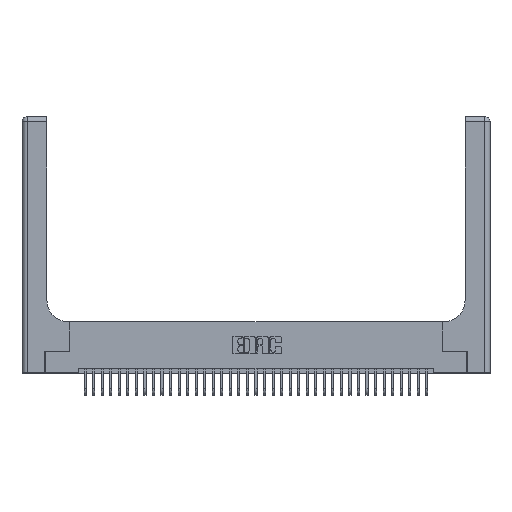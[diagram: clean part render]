
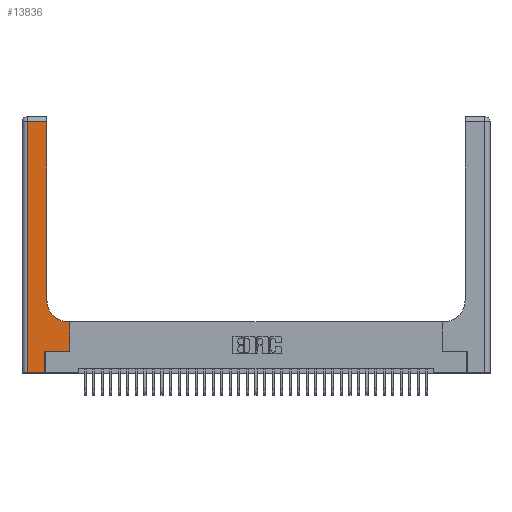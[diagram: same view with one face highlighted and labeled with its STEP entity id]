
A CAD part, top view. The second image highlights one B-rep face of the part: STEP entity #13836.
In plain terms, the highlighted planar face has unit normal (0, 0, 1).
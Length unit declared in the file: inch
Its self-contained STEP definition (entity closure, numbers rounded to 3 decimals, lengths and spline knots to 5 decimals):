
#335 = DIRECTION ( 'NONE',  ( 0., 1., 0. ) ) ;
#1182 = EDGE_LOOP ( 'NONE', ( #3528, #18645, #12930, #21307, #23895, #11593, #5812, #29034, #10288 ) ) ;
#1398 = EDGE_CURVE ( 'NONE', #20830, #19128, #17154, .T. ) ;
#1920 = LINE ( 'NONE', #32527, #17076 ) ;
#3303 = LINE ( 'NONE', #16678, #31379 ) ;
#3528 = ORIENTED_EDGE ( 'NONE', *, *, #5199, .T. ) ;
#5199 = EDGE_CURVE ( 'NONE', #33645, #21898, #26045, .T. ) ;
#5226 = DIRECTION ( 'NONE',  ( 0., -1., 0. ) ) ;
#5538 = VERTEX_POINT ( 'NONE', #17578 ) ;
#5812 = ORIENTED_EDGE ( 'NONE', *, *, #19766, .T. ) ;
#5945 = LINE ( 'NONE', #28538, #26597 ) ;
#6381 = CARTESIAN_POINT ( 'NONE',  ( 0.2915, 2.94, 0.37 ) ) ;
#8155 = DIRECTION ( 'NONE',  ( -1., 0., 0. ) ) ;
#9908 = CARTESIAN_POINT ( 'NONE',  ( 0.5415, 0.85, 0.37 ) ) ;
#10036 = EDGE_CURVE ( 'NONE', #13771, #20830, #5945, .T. ) ;
#10288 = ORIENTED_EDGE ( 'NONE', *, *, #23283, .T. ) ;
#10390 = CARTESIAN_POINT ( 'NONE',  ( 0.2915, 0.6, 0.37 ) ) ;
#11514 = DIRECTION ( 'NONE',  ( 1., 0., 0. ) ) ;
#11593 = ORIENTED_EDGE ( 'NONE', *, *, #1398, .T. ) ;
#12111 = DIRECTION ( 'NONE',  ( 0., 1., 0. ) ) ;
#12151 = VECTOR ( 'NONE', #12111, 39.37008 ) ;
#12765 = DIRECTION ( 'NONE',  ( 1., 0., 0. ) ) ;
#12930 = ORIENTED_EDGE ( 'NONE', *, *, #18725, .T. ) ;
#13298 = CARTESIAN_POINT ( 'NONE',  ( 0.2915, 3., 0.37 ) ) ;
#13396 = CARTESIAN_POINT ( 'NONE',  ( 0.269, 0., 0.37 ) ) ;
#13771 = VERTEX_POINT ( 'NONE', #13396 ) ;
#13836 = ADVANCED_FACE ( 'NONE', ( #15735 ), #35849, .F. ) ;
#14869 = VERTEX_POINT ( 'NONE', #15434 ) ;
#15434 = CARTESIAN_POINT ( 'NONE',  ( 0.06, 2.94, 0.37 ) ) ;
#15702 = EDGE_CURVE ( 'NONE', #5538, #33022, #28567, .T. ) ;
#15735 = FACE_OUTER_BOUND ( 'NONE', #1182, .T. ) ;
#15970 = CIRCLE ( 'NONE', #20518, 0.25 ) ;
#16110 = CARTESIAN_POINT ( 'NONE',  ( 0.06, 0., 0.37 ) ) ;
#16678 = CARTESIAN_POINT ( 'NONE',  ( 0.06, 3., 0.37 ) ) ;
#17076 = VECTOR ( 'NONE', #18669, 39.37008 ) ;
#17154 = LINE ( 'NONE', #28203, #30974 ) ;
#17578 = CARTESIAN_POINT ( 'NONE',  ( 0.5585, 0.6, 0.37 ) ) ;
#18645 = ORIENTED_EDGE ( 'NONE', *, *, #23638, .T. ) ;
#18656 = VECTOR ( 'NONE', #21776, 39.37008 ) ;
#18669 = DIRECTION ( 'NONE',  ( 1., 0., 0. ) ) ;
#18725 = EDGE_CURVE ( 'NONE', #14869, #33354, #3303, .T. ) ;
#19128 = VERTEX_POINT ( 'NONE', #34329 ) ;
#19433 = LINE ( 'NONE', #36202, #33181 ) ;
#19766 = EDGE_CURVE ( 'NONE', #19128, #5538, #33404, .T. ) ;
#19785 = DIRECTION ( 'NONE',  ( -1., 0., 0. ) ) ;
#20518 = AXIS2_PLACEMENT_3D ( 'NONE', #9908, #29420, #12765 ) ;
#20830 = VERTEX_POINT ( 'NONE', #29207 ) ;
#21307 = ORIENTED_EDGE ( 'NONE', *, *, #30677, .T. ) ;
#21776 = DIRECTION ( 'NONE',  ( 0., 1., 0. ) ) ;
#21898 = VERTEX_POINT ( 'NONE', #6381 ) ;
#22865 = CARTESIAN_POINT ( 'NONE',  ( 0.5415, 0.6, 0.37 ) ) ;
#23283 = EDGE_CURVE ( 'NONE', #33022, #33645, #15970, .T. ) ;
#23638 = EDGE_CURVE ( 'NONE', #21898, #14869, #19433, .T. ) ;
#23895 = ORIENTED_EDGE ( 'NONE', *, *, #10036, .T. ) ;
#24396 = DIRECTION ( 'NONE',  ( -1., 0., 0. ) ) ;
#24984 = DIRECTION ( 'NONE',  ( 0., 0., -1. ) ) ;
#26045 = LINE ( 'NONE', #13298, #18656 ) ;
#26312 = AXIS2_PLACEMENT_3D ( 'NONE', #30364, #24984, #8155 ) ;
#26597 = VECTOR ( 'NONE', #335, 39.37008 ) ;
#27701 = VECTOR ( 'NONE', #24396, 39.37008 ) ;
#28203 = CARTESIAN_POINT ( 'NONE',  ( 0.269, 0.25, 0.37 ) ) ;
#28538 = CARTESIAN_POINT ( 'NONE',  ( 0.269, 0., 0.37 ) ) ;
#28567 = LINE ( 'NONE', #10390, #27701 ) ;
#28901 = CARTESIAN_POINT ( 'NONE',  ( 0.2915, 0.85, 0.37 ) ) ;
#29034 = ORIENTED_EDGE ( 'NONE', *, *, #15702, .T. ) ;
#29207 = CARTESIAN_POINT ( 'NONE',  ( 0.269, 0.25, 0.37 ) ) ;
#29420 = DIRECTION ( 'NONE',  ( 0., 0., -1. ) ) ;
#30364 = CARTESIAN_POINT ( 'NONE',  ( 0., 3., 0.37 ) ) ;
#30677 = EDGE_CURVE ( 'NONE', #33354, #13771, #1920, .T. ) ;
#30974 = VECTOR ( 'NONE', #11514, 39.37008 ) ;
#31379 = VECTOR ( 'NONE', #5226, 39.37008 ) ;
#32527 = CARTESIAN_POINT ( 'NONE',  ( 0., 0., 0.37 ) ) ;
#33022 = VERTEX_POINT ( 'NONE', #22865 ) ;
#33181 = VECTOR ( 'NONE', #19785, 39.37008 ) ;
#33354 = VERTEX_POINT ( 'NONE', #16110 ) ;
#33404 = LINE ( 'NONE', #34285, #12151 ) ;
#33645 = VERTEX_POINT ( 'NONE', #28901 ) ;
#34285 = CARTESIAN_POINT ( 'NONE',  ( 0.5585, 0.25, 0.37 ) ) ;
#34329 = CARTESIAN_POINT ( 'NONE',  ( 0.5585, 0.25, 0.37 ) ) ;
#35849 = PLANE ( 'NONE',  #26312 ) ;
#36202 = CARTESIAN_POINT ( 'NONE',  ( 0., 2.94, 0.37 ) ) ;
